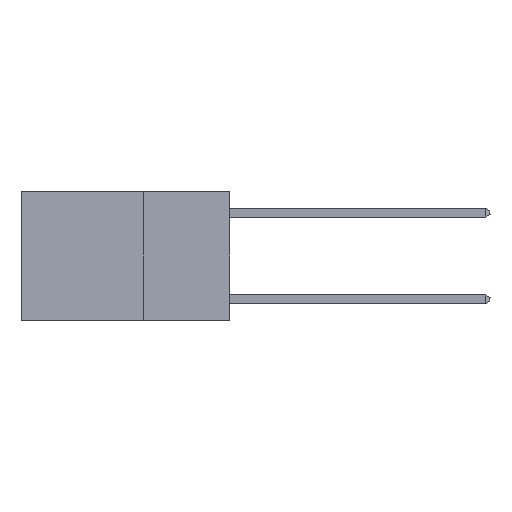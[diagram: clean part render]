
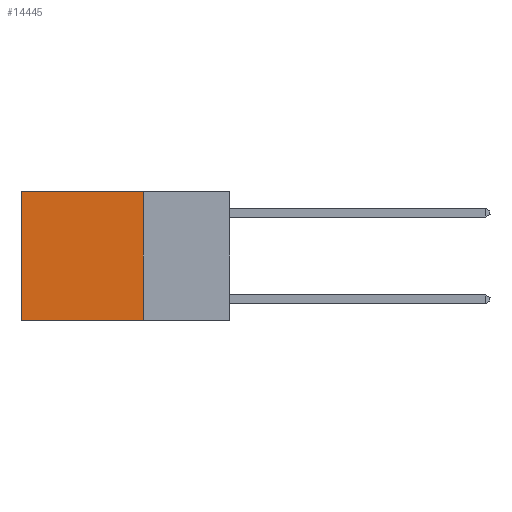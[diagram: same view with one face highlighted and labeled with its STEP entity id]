
A CAD part, left-side view. The second image highlights one B-rep face of the part: STEP entity #14445.
In plain terms, the highlighted planar face has unit normal (-1, 0, 0).
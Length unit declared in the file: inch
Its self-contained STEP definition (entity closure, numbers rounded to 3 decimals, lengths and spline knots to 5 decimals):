
#294 = VECTOR ( 'NONE', #7736, 39.37008 ) ;
#534 = VECTOR ( 'NONE', #10463, 39.37008 ) ;
#888 = ORIENTED_EDGE ( 'NONE', *, *, #8154, .T. ) ;
#1108 = CARTESIAN_POINT ( 'NONE',  ( 0.2625, 0.25, 0. ) ) ;
#2538 = EDGE_CURVE ( 'NONE', #11890, #6363, #7296, .T. ) ;
#3189 = CARTESIAN_POINT ( 'NONE',  ( 0.2625, 0.25, 0. ) ) ;
#3821 = DIRECTION ( 'NONE',  ( 0., 1., 0. ) ) ;
#4258 = LINE ( 'NONE', #8930, #6378 ) ;
#4688 = AXIS2_PLACEMENT_3D ( 'NONE', #3189, #12315, #7830 ) ;
#5052 = CARTESIAN_POINT ( 'NONE',  ( 0.2625, 0.6, 0. ) ) ;
#5072 = ORIENTED_EDGE ( 'NONE', *, *, #14520, .T. ) ;
#5386 = PLANE ( 'NONE',  #4688 ) ;
#5611 = ORIENTED_EDGE ( 'NONE', *, *, #13211, .F. ) ;
#5852 = VERTEX_POINT ( 'NONE', #5052 ) ;
#6363 = VERTEX_POINT ( 'NONE', #10718 ) ;
#6378 = VECTOR ( 'NONE', #13527, 39.37008 ) ;
#6668 = FACE_OUTER_BOUND ( 'NONE', #13023, .T. ) ;
#7090 = LINE ( 'NONE', #12790, #534 ) ;
#7296 = LINE ( 'NONE', #13003, #8525 ) ;
#7578 = LINE ( 'NONE', #10170, #294 ) ;
#7736 = DIRECTION ( 'NONE',  ( 0., 1., 0. ) ) ;
#7830 = DIRECTION ( 'NONE',  ( 0., 0., -1. ) ) ;
#8154 = EDGE_CURVE ( 'NONE', #10498, #5852, #7578, .T. ) ;
#8525 = VECTOR ( 'NONE', #3821, 39.37008 ) ;
#8930 = CARTESIAN_POINT ( 'NONE',  ( 0.2625, 0.6, 0. ) ) ;
#9474 = CARTESIAN_POINT ( 'NONE',  ( 0.2625, 0.25, -0.37 ) ) ;
#10170 = CARTESIAN_POINT ( 'NONE',  ( 0.2625, 0.25, 0. ) ) ;
#10463 = DIRECTION ( 'NONE',  ( 0., 0., -1. ) ) ;
#10498 = VERTEX_POINT ( 'NONE', #1108 ) ;
#10718 = CARTESIAN_POINT ( 'NONE',  ( 0.2625, 0.6, -0.37 ) ) ;
#11154 = ORIENTED_EDGE ( 'NONE', *, *, #2538, .F. ) ;
#11890 = VERTEX_POINT ( 'NONE', #9474 ) ;
#12315 = DIRECTION ( 'NONE',  ( 1., 0., 0. ) ) ;
#12790 = CARTESIAN_POINT ( 'NONE',  ( 0.2625, 0.25, 0. ) ) ;
#13003 = CARTESIAN_POINT ( 'NONE',  ( 0.2625, 0.25, -0.37 ) ) ;
#13023 = EDGE_LOOP ( 'NONE', ( #5072, #11154, #5611, #888 ) ) ;
#13211 = EDGE_CURVE ( 'NONE', #10498, #11890, #7090, .T. ) ;
#13527 = DIRECTION ( 'NONE',  ( 0., 0., -1. ) ) ;
#14445 = ADVANCED_FACE ( 'NONE', ( #6668 ), #5386, .F. ) ;
#14520 = EDGE_CURVE ( 'NONE', #5852, #6363, #4258, .T. ) ;
